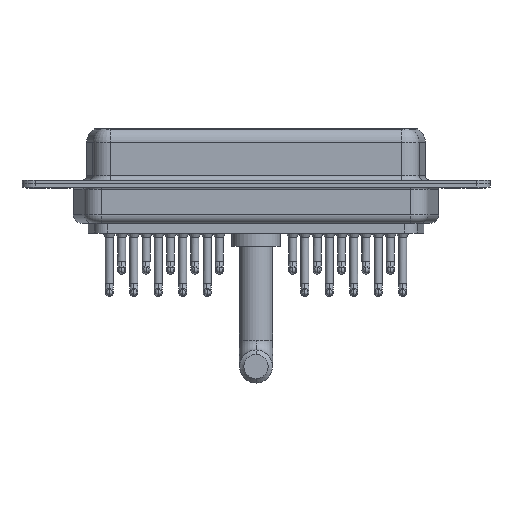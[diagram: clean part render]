
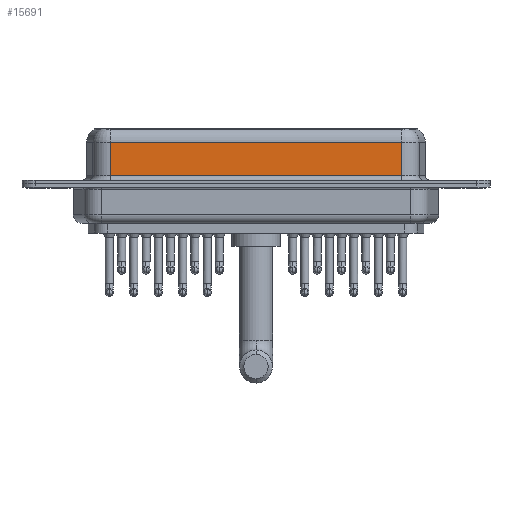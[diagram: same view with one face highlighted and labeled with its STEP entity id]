
A CAD part, front view. The second image highlights one B-rep face of the part: STEP entity #15691.
In plain terms, the highlighted planar face has unit normal (0, -1, 0).
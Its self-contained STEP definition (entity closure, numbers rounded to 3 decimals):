
#780 = DIRECTION ( 'NONE',  ( 0., 0., -1. ) ) ;
#911 = VERTEX_POINT ( 'NONE', #18384 ) ;
#968 = LINE ( 'NONE', #20390, #8262 ) ;
#1057 = EDGE_CURVE ( 'NONE', #3934, #18461, #968, .T. ) ;
#1376 = DIRECTION ( 'NONE',  ( 1., 0., 0. ) ) ;
#1778 = ORIENTED_EDGE ( 'NONE', *, *, #9265, .F. ) ;
#1991 = LINE ( 'NONE', #10425, #3810 ) ;
#2144 = VERTEX_POINT ( 'NONE', #2719 ) ;
#2401 = DIRECTION ( 'NONE',  ( -1., 0., 0. ) ) ;
#2565 = CARTESIAN_POINT ( 'NONE',  ( 7.013, -3.95, 6.4 ) ) ;
#2719 = CARTESIAN_POINT ( 'NONE',  ( 40.037, -3.95, 4.65 ) ) ;
#2937 = ORIENTED_EDGE ( 'NONE', *, *, #20809, .T. ) ;
#3699 = AXIS2_PLACEMENT_3D ( 'NONE', #4809, #19697, #17799 ) ;
#3810 = VECTOR ( 'NONE', #2401, 1000. ) ;
#3934 = VERTEX_POINT ( 'NONE', #6487 ) ;
#4809 = CARTESIAN_POINT ( 'NONE',  ( 40.037, -3.95, 6.4 ) ) ;
#5895 = VECTOR ( 'NONE', #780, 1000. ) ;
#6487 = CARTESIAN_POINT ( 'NONE',  ( 7.013, -3.95, 0.9 ) ) ;
#7981 = PLANE ( 'NONE',  #3699 ) ;
#8262 = VECTOR ( 'NONE', #1376, 1000. ) ;
#9265 = EDGE_CURVE ( 'NONE', #2144, #18461, #10710, .T. ) ;
#10425 = CARTESIAN_POINT ( 'NONE',  ( 40.037, -3.95, 4.65 ) ) ;
#10599 = CARTESIAN_POINT ( 'NONE',  ( 40.037, -3.95, 6.4 ) ) ;
#10609 = ORIENTED_EDGE ( 'NONE', *, *, #1057, .T. ) ;
#10710 = LINE ( 'NONE', #10599, #19033 ) ;
#11071 = EDGE_CURVE ( 'NONE', #911, #3934, #17053, .T. ) ;
#11661 = FACE_OUTER_BOUND ( 'NONE', #14776, .T. ) ;
#13312 = CARTESIAN_POINT ( 'NONE',  ( 40.037, -3.95, 0.9 ) ) ;
#14776 = EDGE_LOOP ( 'NONE', ( #1778, #2937, #16730, #10609 ) ) ;
#15490 = DIRECTION ( 'NONE',  ( 0., 0., -1. ) ) ;
#15691 = ADVANCED_FACE ( 'NONE', ( #11661 ), #7981, .F. ) ;
#16730 = ORIENTED_EDGE ( 'NONE', *, *, #11071, .T. ) ;
#17053 = LINE ( 'NONE', #2565, #5895 ) ;
#17799 = DIRECTION ( 'NONE',  ( 0., 0., 1. ) ) ;
#18384 = CARTESIAN_POINT ( 'NONE',  ( 7.013, -3.95, 4.65 ) ) ;
#18461 = VERTEX_POINT ( 'NONE', #13312 ) ;
#19033 = VECTOR ( 'NONE', #15490, 1000. ) ;
#19697 = DIRECTION ( 'NONE',  ( 0., 1., 0. ) ) ;
#20390 = CARTESIAN_POINT ( 'NONE',  ( 40.037, -3.95, 0.9 ) ) ;
#20809 = EDGE_CURVE ( 'NONE', #2144, #911, #1991, .T. ) ;
